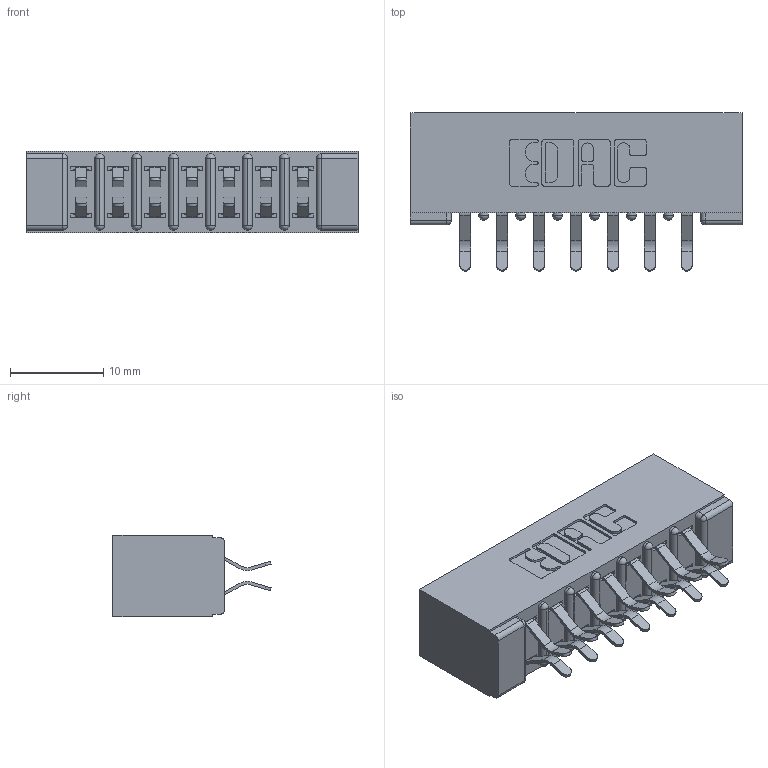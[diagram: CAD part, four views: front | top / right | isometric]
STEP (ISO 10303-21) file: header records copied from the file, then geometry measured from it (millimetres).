
FILE_DESCRIPTION (( 'STEP AP203' ), '1' );
FILE_NAME ('357-014-456-201.STEP', '2020-10-02T18:04:53', ( '' ), ( '' ), 'SwSTEP 2.0', 'SolidWorks 2020', '' );
FILE_SCHEMA (( 'CONFIG_CONTROL_DESIGN' ));
Length unit declared in the file: inch
Products named in the file (3): 357-014-456-201; 307 Part_No Mounting Lugs; 307-290-001_556
Assembly tree (15 placements, depth 2):
  357-014-456-201
    307 Part_No Mounting Lugs
    307-290-001_556  x14
Bounding box: 35.61 x 16.97 x 8.71 mm (x, y, z)
Volume: 2561.6 mm3; surface area: 4198.8 mm2
Topology: 15 solids, 15 shells, 818 faces, 2287 edges, 1482 vertices
Faces by surface type: plane 528, cylinder 274, sphere 16
Entity records: 10366 total; most frequent: CARTESIAN_POINT 1703, DIRECTION 1683, ORIENTED_EDGE 1682, EDGE_CURVE 841, LINE 631, VECTOR 631, VERTEX_POINT 546, AXIS2_PLACEMENT_3D 526
